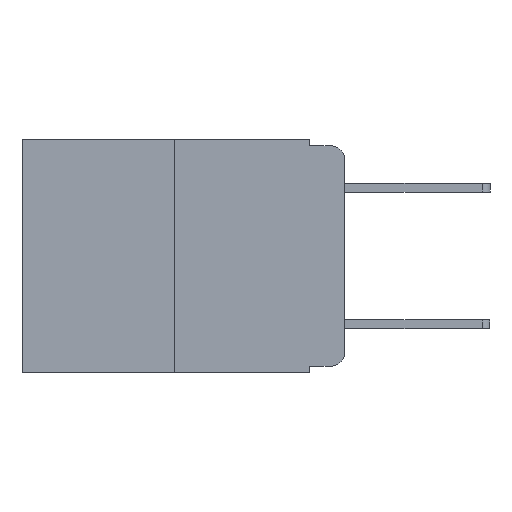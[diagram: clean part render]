
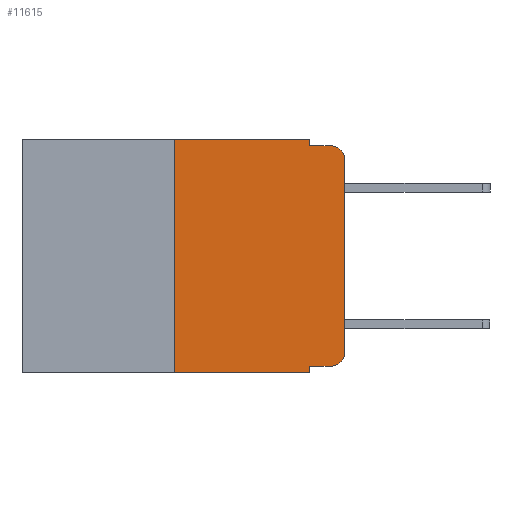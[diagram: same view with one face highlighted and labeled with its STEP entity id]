
A CAD part, left-side view. The second image highlights one B-rep face of the part: STEP entity #11615.
In plain terms, the highlighted planar face has unit normal (-1, 0, 0).
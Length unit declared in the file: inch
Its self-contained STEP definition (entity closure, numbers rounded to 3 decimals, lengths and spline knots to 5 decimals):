
#555 = EDGE_CURVE ( 'NONE', #3387, #11255, #7341, .T. ) ;
#918 = CARTESIAN_POINT ( 'NONE',  ( 0., 0., -0.313 ) ) ;
#1095 = CARTESIAN_POINT ( 'NONE',  ( 0., 0., -0.03 ) ) ;
#1604 = CIRCLE ( 'NONE', #6497, 0.02 ) ;
#2113 = EDGE_CURVE ( 'NONE', #21095, #9458, #16592, .T. ) ;
#2332 = VECTOR ( 'NONE', #8602, 39.37008 ) ;
#2977 = VECTOR ( 'NONE', #13823, 39.37008 ) ;
#3013 = LINE ( 'NONE', #6593, #4110 ) ;
#3387 = VERTEX_POINT ( 'NONE', #5843 ) ;
#3448 = CARTESIAN_POINT ( 'NONE',  ( 0., 0.25, 0. ) ) ;
#3742 = EDGE_CURVE ( 'NONE', #9458, #3387, #15839, .T. ) ;
#3923 = EDGE_LOOP ( 'NONE', ( #8752, #14057, #5063, #6092, #12745, #17055, #5305, #7502, #21949, #15193 ) ) ;
#4110 = VECTOR ( 'NONE', #18500, 39.37008 ) ;
#4179 = CIRCLE ( 'NONE', #17656, 0.02 ) ;
#4221 = CARTESIAN_POINT ( 'NONE',  ( 0., 0.02, -0.313 ) ) ;
#4418 = DIRECTION ( 'NONE',  ( 0., -1., 0. ) ) ;
#4734 = DIRECTION ( 'NONE',  ( 0., -1., 0. ) ) ;
#4759 = PLANE ( 'NONE',  #8961 ) ;
#5063 = ORIENTED_EDGE ( 'NONE', *, *, #555, .F. ) ;
#5117 = VERTEX_POINT ( 'NONE', #918 ) ;
#5163 = LINE ( 'NONE', #14929, #8639 ) ;
#5290 = CARTESIAN_POINT ( 'NONE',  ( 0., 0.02, -0.01 ) ) ;
#5305 = ORIENTED_EDGE ( 'NONE', *, *, #13403, .T. ) ;
#5545 = VECTOR ( 'NONE', #11196, 39.37008 ) ;
#5702 = VECTOR ( 'NONE', #18691, 39.37008 ) ;
#5843 = CARTESIAN_POINT ( 'NONE',  ( 0., 0.051, -0.01 ) ) ;
#5906 = DIRECTION ( 'NONE',  ( 0., 0., -1. ) ) ;
#6092 = ORIENTED_EDGE ( 'NONE', *, *, #3742, .F. ) ;
#6373 = CARTESIAN_POINT ( 'NONE',  ( 0., 0.473, 0. ) ) ;
#6497 = AXIS2_PLACEMENT_3D ( 'NONE', #4221, #16126, #5906 ) ;
#6593 = CARTESIAN_POINT ( 'NONE',  ( 0., 0.051, -0.333 ) ) ;
#7341 = LINE ( 'NONE', #21882, #11337 ) ;
#7502 = ORIENTED_EDGE ( 'NONE', *, *, #10892, .F. ) ;
#8602 = DIRECTION ( 'NONE',  ( 0., 0., 1. ) ) ;
#8639 = VECTOR ( 'NONE', #4734, 39.37008 ) ;
#8752 = ORIENTED_EDGE ( 'NONE', *, *, #14147, .T. ) ;
#8961 = AXIS2_PLACEMENT_3D ( 'NONE', #9843, #9914, #21720 ) ;
#9011 = VERTEX_POINT ( 'NONE', #1095 ) ;
#9458 = VERTEX_POINT ( 'NONE', #10661 ) ;
#9843 = CARTESIAN_POINT ( 'NONE',  ( 0., 0.473, 0. ) ) ;
#9914 = DIRECTION ( 'NONE',  ( 1., 0., 0. ) ) ;
#10107 = CARTESIAN_POINT ( 'NONE',  ( 0., 0.051, 0. ) ) ;
#10661 = CARTESIAN_POINT ( 'NONE',  ( 0., 0.051, 0. ) ) ;
#10727 = VECTOR ( 'NONE', #11784, 39.37008 ) ;
#10768 = VERTEX_POINT ( 'NONE', #19203 ) ;
#10892 = EDGE_CURVE ( 'NONE', #18262, #16838, #19111, .T. ) ;
#11196 = DIRECTION ( 'NONE',  ( 0., 0., -1. ) ) ;
#11255 = VERTEX_POINT ( 'NONE', #5290 ) ;
#11337 = VECTOR ( 'NONE', #4418, 39.37008 ) ;
#11425 = LINE ( 'NONE', #3448, #2332 ) ;
#11574 = DIRECTION ( 'NONE',  ( 0., 0., -1. ) ) ;
#11615 = ADVANCED_FACE ( 'NONE', ( #13785 ), #4759, .F. ) ;
#11784 = DIRECTION ( 'NONE',  ( 0., 0., 1. ) ) ;
#11937 = CARTESIAN_POINT ( 'NONE',  ( 0., 0.051, -0.343 ) ) ;
#12097 = EDGE_CURVE ( 'NONE', #9011, #11255, #4179, .T. ) ;
#12745 = ORIENTED_EDGE ( 'NONE', *, *, #2113, .F. ) ;
#13403 = EDGE_CURVE ( 'NONE', #15392, #16838, #5163, .T. ) ;
#13452 = EDGE_CURVE ( 'NONE', #18262, #10768, #3013, .T. ) ;
#13656 = CARTESIAN_POINT ( 'NONE',  ( 0., 0.25, 0. ) ) ;
#13785 = FACE_OUTER_BOUND ( 'NONE', #3923, .T. ) ;
#13823 = DIRECTION ( 'NONE',  ( 0., -1., 0. ) ) ;
#13935 = CARTESIAN_POINT ( 'NONE',  ( 0., 0.051, -0.333 ) ) ;
#14057 = ORIENTED_EDGE ( 'NONE', *, *, #12097, .T. ) ;
#14147 = EDGE_CURVE ( 'NONE', #5117, #9011, #15250, .T. ) ;
#14531 = CARTESIAN_POINT ( 'NONE',  ( 0., 0.25, -0.343 ) ) ;
#14929 = CARTESIAN_POINT ( 'NONE',  ( 0., 0.473, -0.343 ) ) ;
#15193 = ORIENTED_EDGE ( 'NONE', *, *, #19551, .T. ) ;
#15250 = LINE ( 'NONE', #21878, #10727 ) ;
#15392 = VERTEX_POINT ( 'NONE', #14531 ) ;
#15839 = LINE ( 'NONE', #10107, #5702 ) ;
#16126 = DIRECTION ( 'NONE',  ( -1., 0., 0. ) ) ;
#16592 = LINE ( 'NONE', #6373, #2977 ) ;
#16838 = VERTEX_POINT ( 'NONE', #11937 ) ;
#17055 = ORIENTED_EDGE ( 'NONE', *, *, #21114, .F. ) ;
#17656 = AXIS2_PLACEMENT_3D ( 'NONE', #19666, #18713, #11574 ) ;
#18262 = VERTEX_POINT ( 'NONE', #13935 ) ;
#18500 = DIRECTION ( 'NONE',  ( 0., -1., 0. ) ) ;
#18691 = DIRECTION ( 'NONE',  ( 0., 0., -1. ) ) ;
#18713 = DIRECTION ( 'NONE',  ( -1., 0., 0. ) ) ;
#19111 = LINE ( 'NONE', #19643, #5545 ) ;
#19203 = CARTESIAN_POINT ( 'NONE',  ( 0., 0.02, -0.333 ) ) ;
#19551 = EDGE_CURVE ( 'NONE', #10768, #5117, #1604, .T. ) ;
#19643 = CARTESIAN_POINT ( 'NONE',  ( 0., 0.051, 0. ) ) ;
#19666 = CARTESIAN_POINT ( 'NONE',  ( 0., 0.02, -0.03 ) ) ;
#21095 = VERTEX_POINT ( 'NONE', #13656 ) ;
#21114 = EDGE_CURVE ( 'NONE', #15392, #21095, #11425, .T. ) ;
#21720 = DIRECTION ( 'NONE',  ( 0., 0., -1. ) ) ;
#21878 = CARTESIAN_POINT ( 'NONE',  ( 0., 0., 0. ) ) ;
#21882 = CARTESIAN_POINT ( 'NONE',  ( 0., 0.051, -0.01 ) ) ;
#21949 = ORIENTED_EDGE ( 'NONE', *, *, #13452, .T. ) ;
